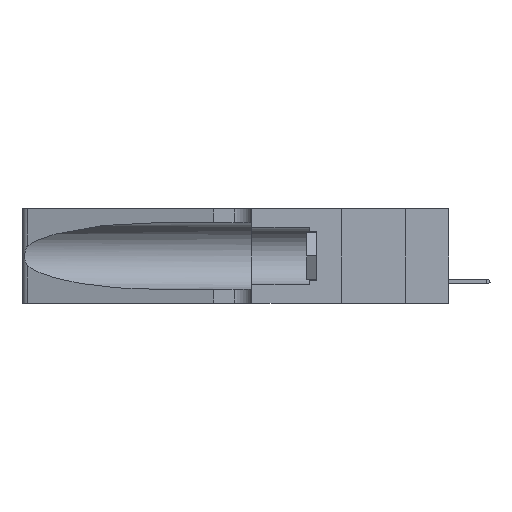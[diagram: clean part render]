
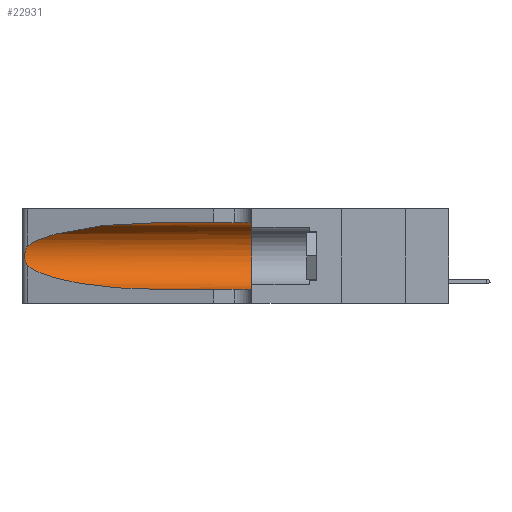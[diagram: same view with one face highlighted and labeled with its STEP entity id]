
A CAD part, left-side view. The second image highlights one B-rep face of the part: STEP entity #22931.
In plain terms, the highlighted cylindrical face has radius 3.308 mm (diameter 6.617 mm), a partial arc.
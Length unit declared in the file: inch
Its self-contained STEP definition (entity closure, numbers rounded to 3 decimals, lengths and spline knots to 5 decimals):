
#293 = CARTESIAN_POINT ( 'NONE',  ( 0.1305, 0.72297, 0.31525 ) ) ;
#621 = EDGE_CURVE ( 'NONE', #2137, #32202, #22780, .T. ) ;
#2137 = VERTEX_POINT ( 'NONE', #36661 ) ;
#2240 = CARTESIAN_POINT ( 'NONE',  ( 0.25487, 1.22718, 0.22369 ) ) ;
#2365 = ORIENTED_EDGE ( 'NONE', *, *, #3551, .T. ) ;
#2724 = CARTESIAN_POINT ( 'NONE',  ( 0.18966, 0.96281, 0.31525 ) ) ;
#3398 = VERTEX_POINT ( 'NONE', #293 ) ;
#3551 = EDGE_CURVE ( 'NONE', #3398, #2137, #35126, .T. ) ;
#3564 = CARTESIAN_POINT ( 'NONE',  ( 0.1305, 1.61858, 0.05475 ) ) ;
#3724 = VECTOR ( 'NONE', #26327, 39.37008 ) ;
#3901 = VERTEX_POINT ( 'NONE', #47632 ) ;
#4362 = EDGE_CURVE ( 'NONE', #3901, #38753, #27921, .T. ) ;
#5253 = ORIENTED_EDGE ( 'NONE', *, *, #621, .T. ) ;
#5488 = CARTESIAN_POINT ( 'NONE',  ( 0.25555, 1.22994, 0.2215 ) ) ;
#5650 = CARTESIAN_POINT ( 'NONE',  ( 0.25639, 1.23184, 0.21858 ) ) ;
#5964 = CARTESIAN_POINT ( 'NONE',  ( 0.25856, 1.23593, 0.16098 ) ) ;
#6499 = DIRECTION ( 'NONE',  ( 0., 0., 1. ) ) ;
#8304 = AXIS2_PLACEMENT_3D ( 'NONE', #36769, #37247, #25789 ) ;
#9399 = CARTESIAN_POINT ( 'NONE',  ( 0.26018, 1.23835, 0.19895 ) ) ;
#10199 = CARTESIAN_POINT ( 'NONE',  ( 0.2373, 1.15595, 0.28018 ) ) ;
#13257 = CARTESIAN_POINT ( 'NONE',  ( 0.26075, 1.23896, 0.19203 ) ) ;
#13566 = LINE ( 'NONE', #3564, #3724 ) ;
#16152 = FACE_OUTER_BOUND ( 'NONE', #24968, .T. ) ;
#17832 = LINE ( 'NONE', #29270, #21928 ) ;
#21476 = CARTESIAN_POINT ( 'NONE',  ( 0.1305, 0.72297, 0.05475 ) ) ;
#21928 = VECTOR ( 'NONE', #22204, 39.37008 ) ;
#22204 = DIRECTION ( 'NONE',  ( 0., -1., 0. ) ) ;
#22711 = ORIENTED_EDGE ( 'NONE', *, *, #44689, .T. ) ;
#22780 = B_SPLINE_CURVE_WITH_KNOTS ( 'NONE', 3,
 ( #2240, #5488, #5650, #32203, #31712, #9399, #13257, #35509, #31871, #5964, #33006, #36309, #35991, #40051 ),
 .UNSPECIFIED., .F., .F.,
 ( 4, 2, 2, 2, 2, 2, 4 ),
 ( 0., 0.00027, 0.00053, 0.00107, 0.0016, 0.00187, 0.00214 ),
 .UNSPECIFIED. ) ;
#22931 = ADVANCED_FACE ( 'NONE', ( #16152 ), #44730, .F. ) ;
#23723 = CARTESIAN_POINT ( 'NONE',  ( 0.1305, 0.35, 0.05475 ) ) ;
#24968 = EDGE_LOOP ( 'NONE', ( #2365, #5253, #22711, #27511, #37982, #26708 ) ) ;
#25789 = DIRECTION ( 'NONE',  ( 0., 0., -1. ) ) ;
#26134 = EDGE_CURVE ( 'NONE', #34161, #38753, #13566, .T. ) ;
#26327 = DIRECTION ( 'NONE',  ( 0., -1., 0. ) ) ;
#26694 = AXIS2_PLACEMENT_3D ( 'NONE', #46851, #28832, #6499 ) ;
#26708 = ORIENTED_EDGE ( 'NONE', *, *, #31009, .F. ) ;
#27511 = ORIENTED_EDGE ( 'NONE', *, *, #26134, .T. ) ;
#27921 = CIRCLE ( 'NONE', #26694, 0.13025 ) ;
#28598 = CARTESIAN_POINT ( 'NONE',  ( 0.1305, 0.72297, 0.31525 ) ) ;
#28832 = DIRECTION ( 'NONE',  ( 0., 1., 0. ) ) ;
#29202 = CARTESIAN_POINT ( 'NONE',  ( 0.1305, 0.72297, 0.05475 ) ) ;
#29270 = CARTESIAN_POINT ( 'NONE',  ( 0.1305, 1.61858, 0.31525 ) ) ;
#29329 = CARTESIAN_POINT ( 'NONE',  ( 0.25487, 1.22718, 0.14631 ) ) ;
#31009 = EDGE_CURVE ( 'NONE', #3398, #3901, #17832, .T. ) ;
#31712 = CARTESIAN_POINT ( 'NONE',  ( 0.25854, 1.2359, 0.20912 ) ) ;
#31871 = CARTESIAN_POINT ( 'NONE',  ( 0.26017, 1.23833, 0.17102 ) ) ;
#32022 = CARTESIAN_POINT ( 'NONE',  ( 0.25487, 1.22718, 0.22369 ) ) ;
#32202 = VERTEX_POINT ( 'NONE', #41087 ) ;
#32203 = CARTESIAN_POINT ( 'NONE',  ( 0.25787, 1.23484, 0.2124 ) ) ;
#33006 = CARTESIAN_POINT ( 'NONE',  ( 0.25789, 1.23486, 0.15765 ) ) ;
#33974 =( BOUNDED_CURVE ( )  B_SPLINE_CURVE ( 3, ( #29329, #40613, #43835, #21476 ),
 .UNSPECIFIED., .F., .F. ) 
 B_SPLINE_CURVE_WITH_KNOTS ( ( 4, 4 ),
 ( 3.44316, 4.71239 ),
 .UNSPECIFIED. ) 
 CURVE ( )  GEOMETRIC_REPRESENTATION_ITEM ( )  RATIONAL_B_SPLINE_CURVE ( ( 1., 0.87, 0.87, 1. ) ) 
 REPRESENTATION_ITEM ( '' )  );
#34161 = VERTEX_POINT ( 'NONE', #29202 ) ;
#35126 =( BOUNDED_CURVE ( )  B_SPLINE_CURVE ( 3, ( #28598, #2724, #10199, #32022 ),
 .UNSPECIFIED., .F., .F. ) 
 B_SPLINE_CURVE_WITH_KNOTS ( ( 4, 4 ),
 ( 1.5708, 2.84003 ),
 .UNSPECIFIED. ) 
 CURVE ( )  GEOMETRIC_REPRESENTATION_ITEM ( )  RATIONAL_B_SPLINE_CURVE ( ( 1., 0.87, 0.87, 1. ) ) 
 REPRESENTATION_ITEM ( '' )  );
#35509 = CARTESIAN_POINT ( 'NONE',  ( 0.26075, 1.23896, 0.178 ) ) ;
#35991 = CARTESIAN_POINT ( 'NONE',  ( 0.25555, 1.22993, 0.14849 ) ) ;
#36309 = CARTESIAN_POINT ( 'NONE',  ( 0.25639, 1.23186, 0.15144 ) ) ;
#36661 = CARTESIAN_POINT ( 'NONE',  ( 0.25487, 1.22718, 0.22369 ) ) ;
#36769 = CARTESIAN_POINT ( 'NONE',  ( 0.1305, 1.61858, 0.185 ) ) ;
#37247 = DIRECTION ( 'NONE',  ( 0., -1., 0. ) ) ;
#37982 = ORIENTED_EDGE ( 'NONE', *, *, #4362, .F. ) ;
#38753 = VERTEX_POINT ( 'NONE', #23723 ) ;
#40051 = CARTESIAN_POINT ( 'NONE',  ( 0.25487, 1.22718, 0.14631 ) ) ;
#40613 = CARTESIAN_POINT ( 'NONE',  ( 0.2373, 1.15595, 0.08982 ) ) ;
#41087 = CARTESIAN_POINT ( 'NONE',  ( 0.25487, 1.22718, 0.14631 ) ) ;
#43835 = CARTESIAN_POINT ( 'NONE',  ( 0.18966, 0.96281, 0.05475 ) ) ;
#44689 = EDGE_CURVE ( 'NONE', #32202, #34161, #33974, .T. ) ;
#44730 = CYLINDRICAL_SURFACE ( 'NONE', #8304, 0.13025 ) ;
#46851 = CARTESIAN_POINT ( 'NONE',  ( 0.1305, 0.35, 0.185 ) ) ;
#47632 = CARTESIAN_POINT ( 'NONE',  ( 0.1305, 0.35, 0.31525 ) ) ;
